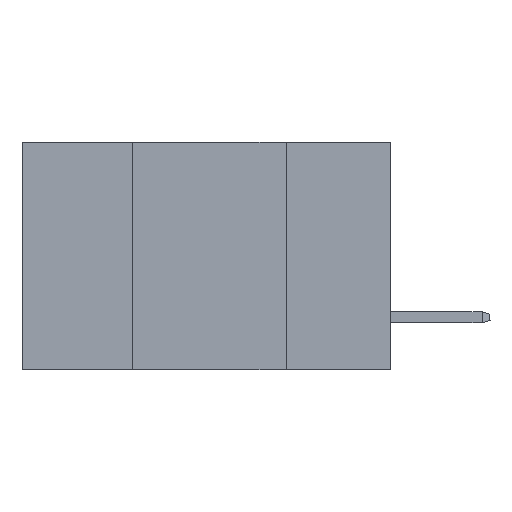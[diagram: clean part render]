
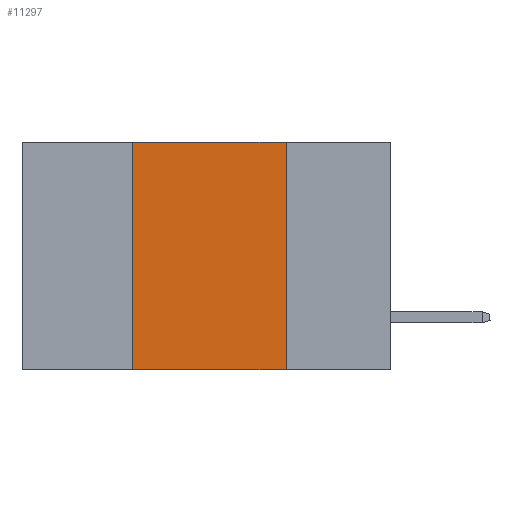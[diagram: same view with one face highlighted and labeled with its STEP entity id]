
A CAD part, left-side view. The second image highlights one B-rep face of the part: STEP entity #11297.
In plain terms, the highlighted planar face has unit normal (-1, 0, 0).
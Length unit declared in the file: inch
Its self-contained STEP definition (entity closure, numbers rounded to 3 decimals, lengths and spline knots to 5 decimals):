
#905 = LINE ( 'NONE', #6084, #1531 ) ;
#1087 = DIRECTION ( 'NONE',  ( 0., 0., 1. ) ) ;
#1531 = VECTOR ( 'NONE', #13340, 39.37008 ) ;
#4075 = PLANE ( 'NONE',  #7925 ) ;
#4219 = DIRECTION ( 'NONE',  ( 0., -1., 0. ) ) ;
#4903 = CARTESIAN_POINT ( 'NONE',  ( 0., 0.42, -0.37 ) ) ;
#5568 = ORIENTED_EDGE ( 'NONE', *, *, #13893, .F. ) ;
#6084 = CARTESIAN_POINT ( 'NONE',  ( 0., 0.6, 0. ) ) ;
#6497 = VECTOR ( 'NONE', #12844, 39.37008 ) ;
#6985 = EDGE_LOOP ( 'NONE', ( #8995, #5568, #8296, #17373 ) ) ;
#7032 = DIRECTION ( 'NONE',  ( 1., 0., 0. ) ) ;
#7117 = CARTESIAN_POINT ( 'NONE',  ( 0., 0.6, -0.37 ) ) ;
#7925 = AXIS2_PLACEMENT_3D ( 'NONE', #15698, #7032, #9969 ) ;
#8296 = ORIENTED_EDGE ( 'NONE', *, *, #11680, .F. ) ;
#8379 = LINE ( 'NONE', #7117, #12859 ) ;
#8995 = ORIENTED_EDGE ( 'NONE', *, *, #11240, .F. ) ;
#9255 = LINE ( 'NONE', #12347, #16257 ) ;
#9969 = DIRECTION ( 'NONE',  ( 0., 0., -1. ) ) ;
#10865 = EDGE_CURVE ( 'NONE', #16409, #14816, #8379, .T. ) ;
#11094 = CARTESIAN_POINT ( 'NONE',  ( 0., 0.17, 0. ) ) ;
#11240 = EDGE_CURVE ( 'NONE', #15858, #14816, #15360, .T. ) ;
#11297 = ADVANCED_FACE ( 'NONE', ( #17401 ), #4075, .F. ) ;
#11670 = VERTEX_POINT ( 'NONE', #13779 ) ;
#11680 = EDGE_CURVE ( 'NONE', #16409, #11670, #9255, .T. ) ;
#12347 = CARTESIAN_POINT ( 'NONE',  ( 0., 0.42, 0. ) ) ;
#12844 = DIRECTION ( 'NONE',  ( 0., 0., -1. ) ) ;
#12859 = VECTOR ( 'NONE', #4219, 39.37008 ) ;
#12967 = CARTESIAN_POINT ( 'NONE',  ( 0., 0.17, 0. ) ) ;
#13340 = DIRECTION ( 'NONE',  ( 0., -1., 0. ) ) ;
#13779 = CARTESIAN_POINT ( 'NONE',  ( 0., 0.42, 0. ) ) ;
#13893 = EDGE_CURVE ( 'NONE', #11670, #15858, #905, .T. ) ;
#14816 = VERTEX_POINT ( 'NONE', #18815 ) ;
#15360 = LINE ( 'NONE', #12967, #6497 ) ;
#15698 = CARTESIAN_POINT ( 'NONE',  ( 0., 0.6, 0. ) ) ;
#15858 = VERTEX_POINT ( 'NONE', #11094 ) ;
#16257 = VECTOR ( 'NONE', #1087, 39.37008 ) ;
#16409 = VERTEX_POINT ( 'NONE', #4903 ) ;
#17373 = ORIENTED_EDGE ( 'NONE', *, *, #10865, .T. ) ;
#17401 = FACE_OUTER_BOUND ( 'NONE', #6985, .T. ) ;
#18815 = CARTESIAN_POINT ( 'NONE',  ( 0., 0.17, -0.37 ) ) ;
